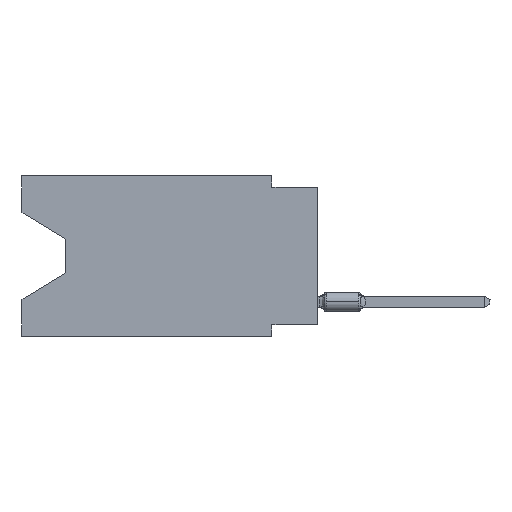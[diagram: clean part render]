
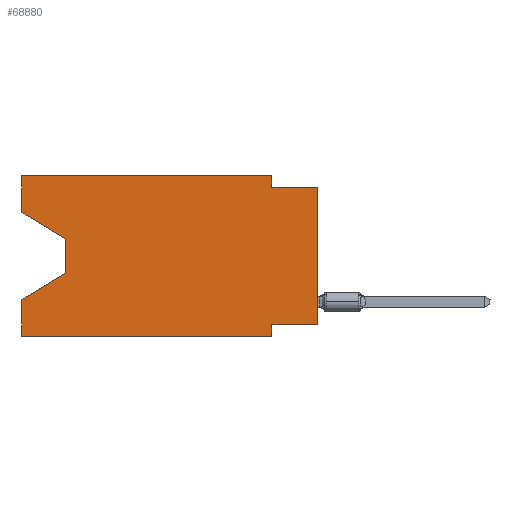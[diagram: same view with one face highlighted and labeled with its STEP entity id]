
A CAD part, left-side view. The second image highlights one B-rep face of the part: STEP entity #68880.
In plain terms, the highlighted planar face has unit normal (-1, 0, 0).
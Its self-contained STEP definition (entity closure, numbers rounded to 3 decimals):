
#226 = DIRECTION ( 'NONE',  ( 0., 0., 1. ) ) ;
#578 = VECTOR ( 'NONE', #226, 1000. ) ;
#909 = LINE ( 'NONE', #12465, #69580 ) ;
#1366 = VERTEX_POINT ( 'NONE', #20565 ) ;
#4026 = CARTESIAN_POINT ( 'NONE',  ( 0., 13.97, -3.505 ) ) ;
#4645 = CARTESIAN_POINT ( 'NONE',  ( 0., 16.383, -8.89 ) ) ;
#4937 = ORIENTED_EDGE ( 'NONE', *, *, #41572, .F. ) ;
#5250 = FACE_OUTER_BOUND ( 'NONE', #55194, .T. ) ;
#6389 = VECTOR ( 'NONE', #43406, 1000. ) ;
#6508 = LINE ( 'NONE', #10927, #6389 ) ;
#6933 = CARTESIAN_POINT ( 'NONE',  ( 0., 16.383, 0. ) ) ;
#7245 = EDGE_CURVE ( 'NONE', #19517, #14511, #68289, .T. ) ;
#7427 = VERTEX_POINT ( 'NONE', #50333 ) ;
#7790 = EDGE_CURVE ( 'NONE', #53961, #1366, #23727, .T. ) ;
#8249 = CARTESIAN_POINT ( 'NONE',  ( 0., 16.383, -8.89 ) ) ;
#8900 = DIRECTION ( 'NONE',  ( 0., 0.855, -0.519 ) ) ;
#10927 = CARTESIAN_POINT ( 'NONE',  ( 0., 13.97, -3.505 ) ) ;
#11738 = CARTESIAN_POINT ( 'NONE',  ( 0., 16.383, -2.038 ) ) ;
#12465 = CARTESIAN_POINT ( 'NONE',  ( 0., 2.54, -8.89 ) ) ;
#12969 = DIRECTION ( 'NONE',  ( 0., -1., 0. ) ) ;
#13713 = VECTOR ( 'NONE', #8900, 1000. ) ;
#13909 = EDGE_CURVE ( 'NONE', #46217, #33338, #52740, .T. ) ;
#14505 = CARTESIAN_POINT ( 'NONE',  ( 0., 13.97, -5.385 ) ) ;
#14511 = VERTEX_POINT ( 'NONE', #74684 ) ;
#14900 = ORIENTED_EDGE ( 'NONE', *, *, #70355, .F. ) ;
#15471 = CARTESIAN_POINT ( 'NONE',  ( 0., 16.383, 0. ) ) ;
#15662 = VECTOR ( 'NONE', #12969, 1000. ) ;
#17057 = VECTOR ( 'NONE', #23314, 1000. ) ;
#19121 = VECTOR ( 'NONE', #64549, 1000. ) ;
#19517 = VERTEX_POINT ( 'NONE', #14505 ) ;
#20466 = EDGE_CURVE ( 'NONE', #58225, #7427, #49259, .T. ) ;
#20565 = CARTESIAN_POINT ( 'NONE',  ( 0., 2.54, -8.255 ) ) ;
#20710 = CARTESIAN_POINT ( 'NONE',  ( 0., 16.383, 0. ) ) ;
#23314 = DIRECTION ( 'NONE',  ( 0., -0.855, -0.519 ) ) ;
#23359 = VECTOR ( 'NONE', #51086, 1000. ) ;
#23727 = LINE ( 'NONE', #37824, #23359 ) ;
#24908 = VECTOR ( 'NONE', #57172, 1000. ) ;
#25535 = CARTESIAN_POINT ( 'NONE',  ( 0., 0., 0. ) ) ;
#29169 = CARTESIAN_POINT ( 'NONE',  ( 0., 16.383, 0. ) ) ;
#30827 = ORIENTED_EDGE ( 'NONE', *, *, #7790, .F. ) ;
#30843 = LINE ( 'NONE', #38503, #19121 ) ;
#30877 = ORIENTED_EDGE ( 'NONE', *, *, #7245, .T. ) ;
#31822 = AXIS2_PLACEMENT_3D ( 'NONE', #6933, #59088, #83891 ) ;
#32567 = DIRECTION ( 'NONE',  ( 0., 0., -1. ) ) ;
#33296 = VERTEX_POINT ( 'NONE', #4026 ) ;
#33338 = VERTEX_POINT ( 'NONE', #42918 ) ;
#33929 = ORIENTED_EDGE ( 'NONE', *, *, #83006, .T. ) ;
#35410 = CARTESIAN_POINT ( 'NONE',  ( 0., 13.97, -5.385 ) ) ;
#37824 = CARTESIAN_POINT ( 'NONE',  ( 0., 0., -8.255 ) ) ;
#38503 = CARTESIAN_POINT ( 'NONE',  ( 0., 2.54, 0. ) ) ;
#41550 = LINE ( 'NONE', #53125, #61999 ) ;
#41572 = EDGE_CURVE ( 'NONE', #7427, #81446, #30843, .T. ) ;
#41575 = VECTOR ( 'NONE', #55217, 1000. ) ;
#42223 = ORIENTED_EDGE ( 'NONE', *, *, #57595, .T. ) ;
#42918 = CARTESIAN_POINT ( 'NONE',  ( 0., 2.54, -8.89 ) ) ;
#43406 = DIRECTION ( 'NONE',  ( 0., 0., -1. ) ) ;
#44461 = VERTEX_POINT ( 'NONE', #80432 ) ;
#45666 = EDGE_CURVE ( 'NONE', #81446, #44461, #41550, .T. ) ;
#46217 = VERTEX_POINT ( 'NONE', #4645 ) ;
#48283 = CARTESIAN_POINT ( 'NONE',  ( 0., 16.383, 0. ) ) ;
#49259 = LINE ( 'NONE', #29169, #77689 ) ;
#50333 = CARTESIAN_POINT ( 'NONE',  ( 0., 2.54, 0. ) ) ;
#51086 = DIRECTION ( 'NONE',  ( 0., 1., 0. ) ) ;
#52061 = CARTESIAN_POINT ( 'NONE',  ( 0., 2.54, -0.635 ) ) ;
#52740 = LINE ( 'NONE', #8249, #15662 ) ;
#53125 = CARTESIAN_POINT ( 'NONE',  ( 0., 0., -0.635 ) ) ;
#53961 = VERTEX_POINT ( 'NONE', #56448 ) ;
#54801 = LINE ( 'NONE', #15471, #41575 ) ;
#55194 = EDGE_LOOP ( 'NONE', ( #59474, #42223, #30877, #78909, #55633, #79123, #30827, #33929, #59604, #4937, #84156, #14900 ) ) ;
#55217 = DIRECTION ( 'NONE',  ( 0., 0., 1. ) ) ;
#55633 = ORIENTED_EDGE ( 'NONE', *, *, #13909, .T. ) ;
#56066 = EDGE_CURVE ( 'NONE', #82894, #33296, #81872, .T. ) ;
#56448 = CARTESIAN_POINT ( 'NONE',  ( 0., 0., -8.255 ) ) ;
#57172 = DIRECTION ( 'NONE',  ( 0., 0., 1. ) ) ;
#57595 = EDGE_CURVE ( 'NONE', #33296, #19517, #6508, .T. ) ;
#58020 = LINE ( 'NONE', #25535, #24908 ) ;
#58225 = VERTEX_POINT ( 'NONE', #48283 ) ;
#58667 = PLANE ( 'NONE',  #31822 ) ;
#59088 = DIRECTION ( 'NONE',  ( 1., 0., 0. ) ) ;
#59474 = ORIENTED_EDGE ( 'NONE', *, *, #56066, .T. ) ;
#59604 = ORIENTED_EDGE ( 'NONE', *, *, #45666, .F. ) ;
#61999 = VECTOR ( 'NONE', #80860, 1000. ) ;
#62998 = EDGE_CURVE ( 'NONE', #1366, #33338, #909, .T. ) ;
#64549 = DIRECTION ( 'NONE',  ( 0., 0., -1. ) ) ;
#65166 = LINE ( 'NONE', #20710, #578 ) ;
#68289 = LINE ( 'NONE', #35410, #13713 ) ;
#68880 = ADVANCED_FACE ( 'NONE', ( #5250 ), #58667, .F. ) ;
#69580 = VECTOR ( 'NONE', #32567, 1000. ) ;
#69744 = EDGE_CURVE ( 'NONE', #46217, #14511, #65166, .T. ) ;
#70355 = EDGE_CURVE ( 'NONE', #82894, #58225, #54801, .T. ) ;
#74684 = CARTESIAN_POINT ( 'NONE',  ( 0., 16.383, -6.852 ) ) ;
#77689 = VECTOR ( 'NONE', #82127, 1000. ) ;
#78909 = ORIENTED_EDGE ( 'NONE', *, *, #69744, .F. ) ;
#79123 = ORIENTED_EDGE ( 'NONE', *, *, #62998, .F. ) ;
#80432 = CARTESIAN_POINT ( 'NONE',  ( 0., 0., -0.635 ) ) ;
#80860 = DIRECTION ( 'NONE',  ( 0., -1., 0. ) ) ;
#81153 = CARTESIAN_POINT ( 'NONE',  ( 0., 16.383, -2.038 ) ) ;
#81446 = VERTEX_POINT ( 'NONE', #52061 ) ;
#81872 = LINE ( 'NONE', #11738, #17057 ) ;
#82127 = DIRECTION ( 'NONE',  ( 0., -1., 0. ) ) ;
#82894 = VERTEX_POINT ( 'NONE', #81153 ) ;
#83006 = EDGE_CURVE ( 'NONE', #53961, #44461, #58020, .T. ) ;
#83891 = DIRECTION ( 'NONE',  ( 0., 0., -1. ) ) ;
#84156 = ORIENTED_EDGE ( 'NONE', *, *, #20466, .F. ) ;
